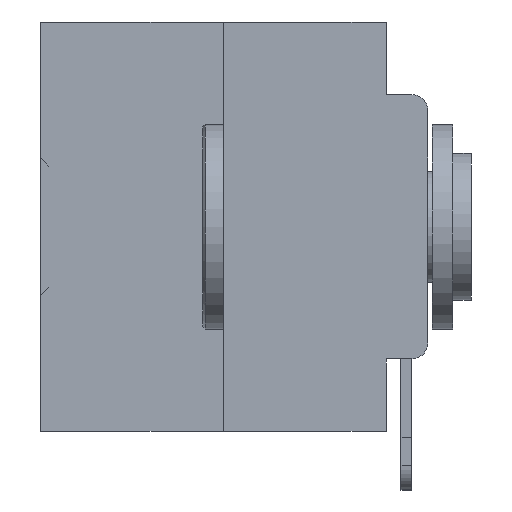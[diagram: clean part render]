
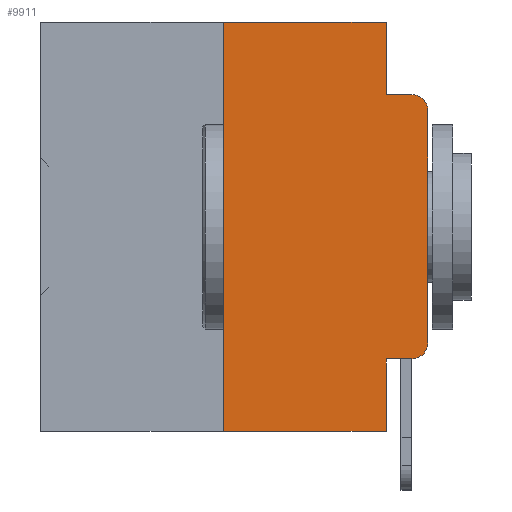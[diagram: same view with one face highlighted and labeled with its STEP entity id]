
A CAD part, left-side view. The second image highlights one B-rep face of the part: STEP entity #9911.
In plain terms, the highlighted planar face has unit normal (-1, 0, 0).
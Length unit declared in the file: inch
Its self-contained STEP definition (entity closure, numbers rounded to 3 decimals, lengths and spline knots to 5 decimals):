
#56 = VECTOR ( 'NONE', #3842, 39.37008 ) ;
#120 = DIRECTION ( 'NONE',  ( 0., -1., 0. ) ) ;
#473 = CARTESIAN_POINT ( 'NONE',  ( 0., 0.25, 0. ) ) ;
#1216 = EDGE_CURVE ( 'NONE', #5422, #21946, #9536, .T. ) ;
#1319 = ORIENTED_EDGE ( 'NONE', *, *, #35145, .F. ) ;
#1911 = DIRECTION ( 'NONE',  ( 0., -1., 0. ) ) ;
#3154 = EDGE_CURVE ( 'NONE', #13837, #22734, #16843, .T. ) ;
#3226 = VERTEX_POINT ( 'NONE', #3537 ) ;
#3401 = DIRECTION ( 'NONE',  ( 1., 0., 0. ) ) ;
#3537 = CARTESIAN_POINT ( 'NONE',  ( 0., 0., -0.1085 ) ) ;
#3842 = DIRECTION ( 'NONE',  ( 0., -1., 0. ) ) ;
#4179 = VERTEX_POINT ( 'NONE', #24778 ) ;
#5422 = VERTEX_POINT ( 'NONE', #23633 ) ;
#5482 = VECTOR ( 'NONE', #120, 39.37008 ) ;
#6259 = PLANE ( 'NONE',  #8973 ) ;
#6490 = LINE ( 'NONE', #473, #29502 ) ;
#6614 = CARTESIAN_POINT ( 'NONE',  ( 0., 0.02, -0.3915 ) ) ;
#6692 = CARTESIAN_POINT ( 'NONE',  ( 0., 0., -0.3915 ) ) ;
#7225 = CARTESIAN_POINT ( 'NONE',  ( 0., 0.051, -0.0885 ) ) ;
#7690 = VECTOR ( 'NONE', #8739, 39.37008 ) ;
#8680 = EDGE_CURVE ( 'NONE', #3226, #22734, #24046, .T. ) ;
#8739 = DIRECTION ( 'NONE',  ( 0., 0., 1. ) ) ;
#8765 = CARTESIAN_POINT ( 'NONE',  ( 0., 0.25, 0. ) ) ;
#8827 = DIRECTION ( 'NONE',  ( -1., 0., 0. ) ) ;
#8917 = CARTESIAN_POINT ( 'NONE',  ( 0., 0.051, -0.5 ) ) ;
#8973 = AXIS2_PLACEMENT_3D ( 'NONE', #12267, #3401, #24326 ) ;
#9536 = LINE ( 'NONE', #35439, #38596 ) ;
#9617 = DIRECTION ( 'NONE',  ( 0., 0., -1. ) ) ;
#9653 = ORIENTED_EDGE ( 'NONE', *, *, #8680, .T. ) ;
#9687 = ORIENTED_EDGE ( 'NONE', *, *, #31294, .T. ) ;
#9844 = VECTOR ( 'NONE', #25451, 39.37008 ) ;
#9911 = ADVANCED_FACE ( 'NONE', ( #12282 ), #6259, .F. ) ;
#10581 = ORIENTED_EDGE ( 'NONE', *, *, #3154, .F. ) ;
#10779 = LINE ( 'NONE', #31377, #9844 ) ;
#11577 = ORIENTED_EDGE ( 'NONE', *, *, #29798, .T. ) ;
#12267 = CARTESIAN_POINT ( 'NONE',  ( 0., 0.473, 0. ) ) ;
#12282 = FACE_OUTER_BOUND ( 'NONE', #20638, .T. ) ;
#12686 = VERTEX_POINT ( 'NONE', #29039 ) ;
#12779 = CARTESIAN_POINT ( 'NONE',  ( 0., 0.051, 0. ) ) ;
#12975 = EDGE_CURVE ( 'NONE', #5422, #24950, #6490, .T. ) ;
#13085 = LINE ( 'NONE', #25886, #36117 ) ;
#13412 = LINE ( 'NONE', #17989, #5482 ) ;
#13837 = VERTEX_POINT ( 'NONE', #35315 ) ;
#14078 = DIRECTION ( 'NONE',  ( 0., 0., -1. ) ) ;
#15147 = CIRCLE ( 'NONE', #20434, 0.02 ) ;
#15584 = LINE ( 'NONE', #29760, #7690 ) ;
#15907 = VERTEX_POINT ( 'NONE', #6692 ) ;
#16649 = ORIENTED_EDGE ( 'NONE', *, *, #18720, .T. ) ;
#16684 = ORIENTED_EDGE ( 'NONE', *, *, #34576, .F. ) ;
#16843 = LINE ( 'NONE', #7225, #56 ) ;
#17989 = CARTESIAN_POINT ( 'NONE',  ( 0., 0.051, -0.4115 ) ) ;
#18720 = EDGE_CURVE ( 'NONE', #15907, #3226, #15584, .T. ) ;
#18729 = AXIS2_PLACEMENT_3D ( 'NONE', #26790, #8827, #29839 ) ;
#20434 = AXIS2_PLACEMENT_3D ( 'NONE', #6614, #27615, #9617 ) ;
#20638 = EDGE_LOOP ( 'NONE', ( #16649, #9653, #10581, #1319, #33164, #27051, #22829, #16684, #9687, #11577 ) ) ;
#21946 = VERTEX_POINT ( 'NONE', #8917 ) ;
#22734 = VERTEX_POINT ( 'NONE', #31060 ) ;
#22829 = ORIENTED_EDGE ( 'NONE', *, *, #1216, .T. ) ;
#23633 = CARTESIAN_POINT ( 'NONE',  ( 0., 0.25, -0.5 ) ) ;
#24046 = CIRCLE ( 'NONE', #18729, 0.02 ) ;
#24326 = DIRECTION ( 'NONE',  ( 0., 0., -1. ) ) ;
#24778 = CARTESIAN_POINT ( 'NONE',  ( 0., 0.051, -0.4115 ) ) ;
#24950 = VERTEX_POINT ( 'NONE', #8765 ) ;
#25451 = DIRECTION ( 'NONE',  ( 0., -1., 0. ) ) ;
#25886 = CARTESIAN_POINT ( 'NONE',  ( 0., 0.051, 0. ) ) ;
#26776 = LINE ( 'NONE', #29096, #27754 ) ;
#26790 = CARTESIAN_POINT ( 'NONE',  ( 0., 0.02, -0.1085 ) ) ;
#27051 = ORIENTED_EDGE ( 'NONE', *, *, #12975, .F. ) ;
#27615 = DIRECTION ( 'NONE',  ( -1., 0., 0. ) ) ;
#27754 = VECTOR ( 'NONE', #14078, 39.37008 ) ;
#29039 = CARTESIAN_POINT ( 'NONE',  ( 0., 0.02, -0.4115 ) ) ;
#29096 = CARTESIAN_POINT ( 'NONE',  ( 0., 0.051, 0. ) ) ;
#29186 = VERTEX_POINT ( 'NONE', #12779 ) ;
#29502 = VECTOR ( 'NONE', #30467, 39.37008 ) ;
#29760 = CARTESIAN_POINT ( 'NONE',  ( 0., 0., 0. ) ) ;
#29798 = EDGE_CURVE ( 'NONE', #12686, #15907, #15147, .T. ) ;
#29839 = DIRECTION ( 'NONE',  ( 0., 0., -1. ) ) ;
#30467 = DIRECTION ( 'NONE',  ( 0., 0., 1. ) ) ;
#31060 = CARTESIAN_POINT ( 'NONE',  ( 0., 0.02, -0.0885 ) ) ;
#31294 = EDGE_CURVE ( 'NONE', #4179, #12686, #13412, .T. ) ;
#31377 = CARTESIAN_POINT ( 'NONE',  ( 0., 0.473, 0. ) ) ;
#31941 = DIRECTION ( 'NONE',  ( 0., 0., -1. ) ) ;
#33164 = ORIENTED_EDGE ( 'NONE', *, *, #35731, .F. ) ;
#34576 = EDGE_CURVE ( 'NONE', #4179, #21946, #26776, .T. ) ;
#35145 = EDGE_CURVE ( 'NONE', #29186, #13837, #13085, .T. ) ;
#35315 = CARTESIAN_POINT ( 'NONE',  ( 0., 0.051, -0.0885 ) ) ;
#35439 = CARTESIAN_POINT ( 'NONE',  ( 0., 0.473, -0.5 ) ) ;
#35731 = EDGE_CURVE ( 'NONE', #24950, #29186, #10779, .T. ) ;
#36117 = VECTOR ( 'NONE', #31941, 39.37008 ) ;
#38596 = VECTOR ( 'NONE', #1911, 39.37008 ) ;
